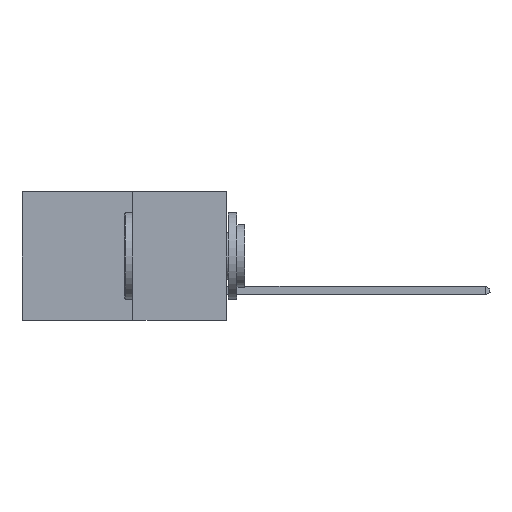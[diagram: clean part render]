
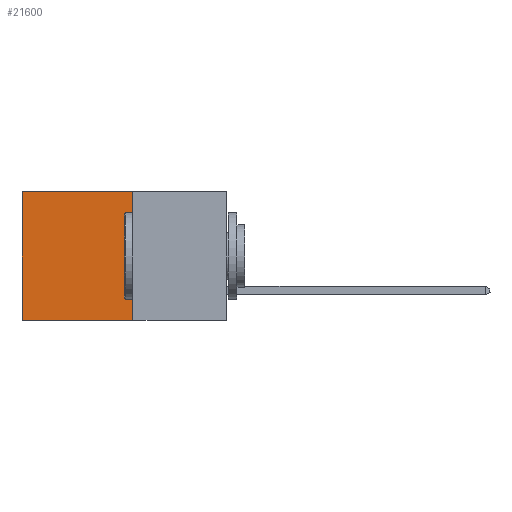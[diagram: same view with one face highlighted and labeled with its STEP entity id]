
A CAD part, left-side view. The second image highlights one B-rep face of the part: STEP entity #21600.
In plain terms, the highlighted planar face has unit normal (-1, 0, 0).
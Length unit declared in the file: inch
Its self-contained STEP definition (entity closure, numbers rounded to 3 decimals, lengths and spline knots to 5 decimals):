
#326 = LINE ( 'NONE', #10299, #24179 ) ;
#722 = EDGE_CURVE ( 'NONE', #7360, #21200, #28266, .T. ) ;
#2178 = ORIENTED_EDGE ( 'NONE', *, *, #9795, .F. ) ;
#2252 = DIRECTION ( 'NONE',  ( 0., 1., 0. ) ) ;
#5750 = CARTESIAN_POINT ( 'NONE',  ( 0.277, 0.59, -0.37 ) ) ;
#5822 = CARTESIAN_POINT ( 'NONE',  ( 0.277, 0.59, -0.37 ) ) ;
#6261 = ORIENTED_EDGE ( 'NONE', *, *, #11478, .T. ) ;
#6361 = VECTOR ( 'NONE', #21433, 39.37008 ) ;
#7074 = CARTESIAN_POINT ( 'NONE',  ( 0.277, 0.27, -0.37 ) ) ;
#7360 = VERTEX_POINT ( 'NONE', #17548 ) ;
#9734 = FACE_OUTER_BOUND ( 'NONE', #16690, .T. ) ;
#9795 = EDGE_CURVE ( 'NONE', #19638, #11805, #326, .T. ) ;
#9979 = VECTOR ( 'NONE', #13737, 39.37008 ) ;
#10299 = CARTESIAN_POINT ( 'NONE',  ( 0.277, 0.27, -0.37 ) ) ;
#11478 = EDGE_CURVE ( 'NONE', #19638, #7360, #14767, .T. ) ;
#11632 = PLANE ( 'NONE',  #19720 ) ;
#11740 = DIRECTION ( 'NONE',  ( 1., 0., 0. ) ) ;
#11805 = VERTEX_POINT ( 'NONE', #22882 ) ;
#13385 = EDGE_CURVE ( 'NONE', #11805, #21200, #18644, .T. ) ;
#13737 = DIRECTION ( 'NONE',  ( 0., 0., -1. ) ) ;
#13855 = CARTESIAN_POINT ( 'NONE',  ( 0.277, 0.27, 0. ) ) ;
#13955 = CARTESIAN_POINT ( 'NONE',  ( 0.277, 0.27, 0. ) ) ;
#14067 = VECTOR ( 'NONE', #2252, 39.37008 ) ;
#14767 = LINE ( 'NONE', #13855, #14067 ) ;
#16690 = EDGE_LOOP ( 'NONE', ( #19462, #17899, #2178, #6261 ) ) ;
#17548 = CARTESIAN_POINT ( 'NONE',  ( 0.277, 0.59, 0. ) ) ;
#17899 = ORIENTED_EDGE ( 'NONE', *, *, #13385, .F. ) ;
#18644 = LINE ( 'NONE', #19107, #6361 ) ;
#19107 = CARTESIAN_POINT ( 'NONE',  ( 0.277, 0.27, -0.37 ) ) ;
#19462 = ORIENTED_EDGE ( 'NONE', *, *, #722, .T. ) ;
#19638 = VERTEX_POINT ( 'NONE', #13955 ) ;
#19720 = AXIS2_PLACEMENT_3D ( 'NONE', #7074, #11740, #27739 ) ;
#21200 = VERTEX_POINT ( 'NONE', #5750 ) ;
#21433 = DIRECTION ( 'NONE',  ( 0., 1., 0. ) ) ;
#21600 = ADVANCED_FACE ( 'NONE', ( #9734 ), #11632, .F. ) ;
#22882 = CARTESIAN_POINT ( 'NONE',  ( 0.277, 0.27, -0.37 ) ) ;
#24179 = VECTOR ( 'NONE', #28715, 39.37008 ) ;
#27739 = DIRECTION ( 'NONE',  ( 0., 0., -1. ) ) ;
#28266 = LINE ( 'NONE', #5822, #9979 ) ;
#28715 = DIRECTION ( 'NONE',  ( 0., 0., -1. ) ) ;
